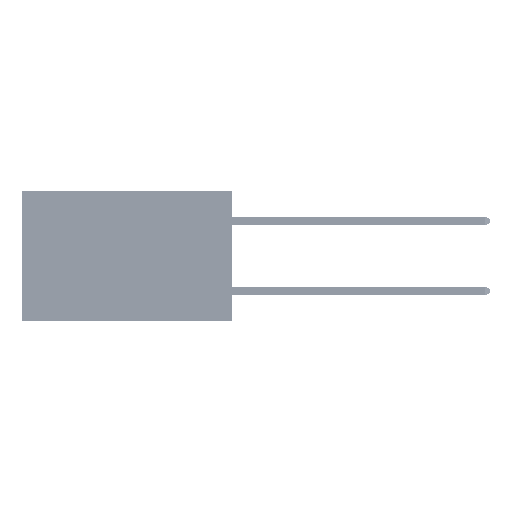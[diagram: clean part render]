
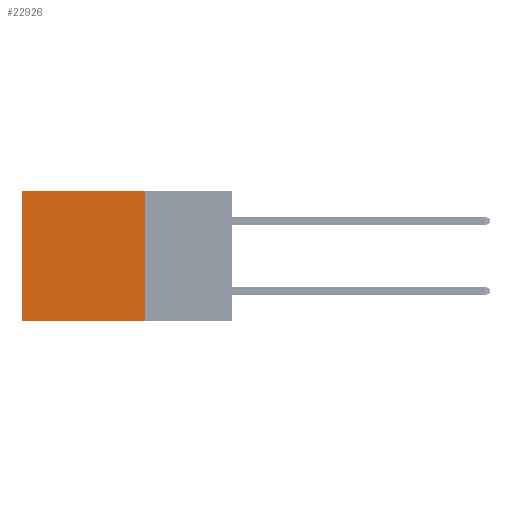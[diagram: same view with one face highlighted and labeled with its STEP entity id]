
A CAD part, left-side view. The second image highlights one B-rep face of the part: STEP entity #22926.
In plain terms, the highlighted planar face has unit normal (-1, 0, 0).
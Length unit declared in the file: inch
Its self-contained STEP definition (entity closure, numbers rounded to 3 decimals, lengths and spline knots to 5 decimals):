
#1620 = VECTOR ( 'NONE', #27867, 39.37008 ) ;
#2725 = CARTESIAN_POINT ( 'NONE',  ( 0.2875, 0.25, 0. ) ) ;
#3187 = PLANE ( 'NONE',  #6192 ) ;
#5001 = CARTESIAN_POINT ( 'NONE',  ( 0.2875, 0.6, -0.37 ) ) ;
#5196 = FACE_OUTER_BOUND ( 'NONE', #22598, .T. ) ;
#5287 = CARTESIAN_POINT ( 'NONE',  ( 0.2875, 0.6, 0. ) ) ;
#6192 = AXIS2_PLACEMENT_3D ( 'NONE', #42609, #34694, #23119 ) ;
#8567 = LINE ( 'NONE', #48781, #45720 ) ;
#8688 = EDGE_CURVE ( 'NONE', #41198, #32004, #47384, .T. ) ;
#9849 = ORIENTED_EDGE ( 'NONE', *, *, #8688, .T. ) ;
#10051 = VERTEX_POINT ( 'NONE', #41320 ) ;
#13198 = VERTEX_POINT ( 'NONE', #31986 ) ;
#14048 = DIRECTION ( 'NONE',  ( 0., 1., 0. ) ) ;
#14911 = EDGE_CURVE ( 'NONE', #10051, #13198, #32621, .T. ) ;
#15194 = ORIENTED_EDGE ( 'NONE', *, *, #50116, .F. ) ;
#18977 = VECTOR ( 'NONE', #33716, 39.37008 ) ;
#22598 = EDGE_LOOP ( 'NONE', ( #9849, #15194, #44583, #37746 ) ) ;
#22926 = ADVANCED_FACE ( 'NONE', ( #5196 ), #3187, .F. ) ;
#23119 = DIRECTION ( 'NONE',  ( 0., 0., -1. ) ) ;
#25160 = EDGE_CURVE ( 'NONE', #10051, #41198, #41809, .T. ) ;
#26984 = VECTOR ( 'NONE', #40615, 39.37008 ) ;
#27867 = DIRECTION ( 'NONE',  ( 0., 1., 0. ) ) ;
#31986 = CARTESIAN_POINT ( 'NONE',  ( 0.2875, 0.25, -0.37 ) ) ;
#32004 = VERTEX_POINT ( 'NONE', #5001 ) ;
#32621 = LINE ( 'NONE', #2725, #18977 ) ;
#32665 = CARTESIAN_POINT ( 'NONE',  ( 0.2875, 0.6, 0. ) ) ;
#33716 = DIRECTION ( 'NONE',  ( 0., 0., -1. ) ) ;
#34694 = DIRECTION ( 'NONE',  ( 1., 0., 0. ) ) ;
#37746 = ORIENTED_EDGE ( 'NONE', *, *, #25160, .T. ) ;
#39424 = CARTESIAN_POINT ( 'NONE',  ( 0.2875, 0.25, 0. ) ) ;
#40615 = DIRECTION ( 'NONE',  ( 0., 0., -1. ) ) ;
#41198 = VERTEX_POINT ( 'NONE', #5287 ) ;
#41320 = CARTESIAN_POINT ( 'NONE',  ( 0.2875, 0.25, 0. ) ) ;
#41809 = LINE ( 'NONE', #39424, #1620 ) ;
#42609 = CARTESIAN_POINT ( 'NONE',  ( 0.2875, 0.25, 0. ) ) ;
#44583 = ORIENTED_EDGE ( 'NONE', *, *, #14911, .F. ) ;
#45720 = VECTOR ( 'NONE', #14048, 39.37008 ) ;
#47384 = LINE ( 'NONE', #32665, #26984 ) ;
#48781 = CARTESIAN_POINT ( 'NONE',  ( 0.2875, 0.25, -0.37 ) ) ;
#50116 = EDGE_CURVE ( 'NONE', #13198, #32004, #8567, .T. ) ;
